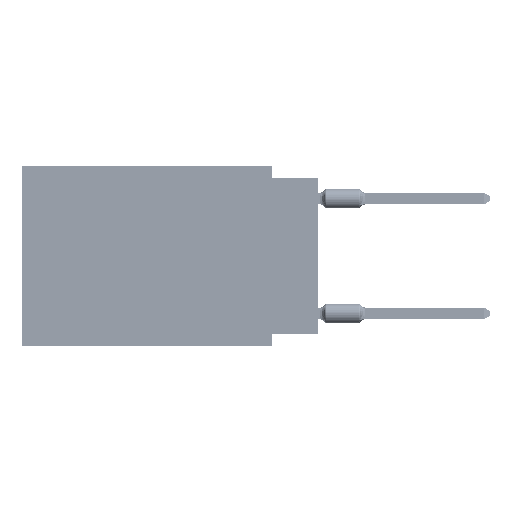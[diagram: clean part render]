
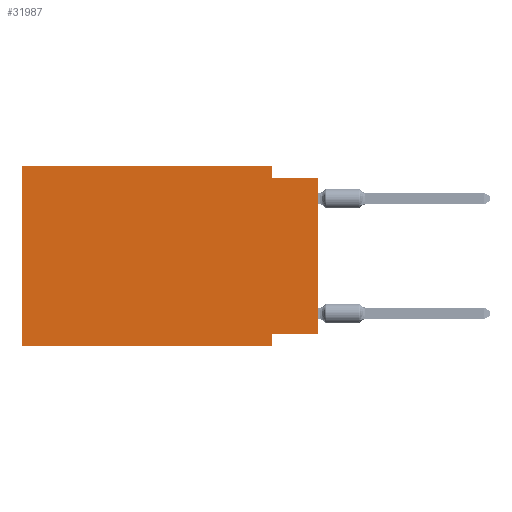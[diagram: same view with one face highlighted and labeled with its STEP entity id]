
A CAD part, left-side view. The second image highlights one B-rep face of the part: STEP entity #31987.
In plain terms, the highlighted planar face has unit normal (-1, 0, 0).
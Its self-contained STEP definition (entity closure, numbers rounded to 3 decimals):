
#2142 = DIRECTION ( 'NONE',  ( 0., 0., -1. ) ) ;
#2933 = LINE ( 'NONE', #9853, #9572 ) ;
#3433 = CARTESIAN_POINT ( 'NONE',  ( 0., 2.54, -9.906 ) ) ;
#5946 = CARTESIAN_POINT ( 'NONE',  ( 0., 0., -9.271 ) ) ;
#6970 = DIRECTION ( 'NONE',  ( 0., -1., 0. ) ) ;
#9033 = VECTOR ( 'NONE', #6970, 1000. ) ;
#9572 = VECTOR ( 'NONE', #56787, 1000. ) ;
#9853 = CARTESIAN_POINT ( 'NONE',  ( 0., 2.54, 0. ) ) ;
#11169 = ORIENTED_EDGE ( 'NONE', *, *, #62654, .F. ) ;
#13111 = VERTEX_POINT ( 'NONE', #47564 ) ;
#13488 = VERTEX_POINT ( 'NONE', #39806 ) ;
#14070 = CARTESIAN_POINT ( 'NONE',  ( 0., 16.383, 0. ) ) ;
#14077 = DIRECTION ( 'NONE',  ( 0., 0., 1. ) ) ;
#14578 = VERTEX_POINT ( 'NONE', #74427 ) ;
#16044 = VECTOR ( 'NONE', #14077, 1000. ) ;
#18585 = DIRECTION ( 'NONE',  ( 0., 0., -1. ) ) ;
#19971 = VECTOR ( 'NONE', #46344, 1000. ) ;
#21335 = VECTOR ( 'NONE', #18585, 1000. ) ;
#21376 = EDGE_CURVE ( 'NONE', #34363, #13488, #2933, .T. ) ;
#21676 = EDGE_LOOP ( 'NONE', ( #48478, #57148, #29792, #11169, #43260, #27646, #43358, #52136 ) ) ;
#22428 = EDGE_CURVE ( 'NONE', #27074, #14578, #39434, .T. ) ;
#22665 = VECTOR ( 'NONE', #39782, 1000. ) ;
#23247 = LINE ( 'NONE', #64027, #19971 ) ;
#24617 = EDGE_CURVE ( 'NONE', #31008, #13111, #66787, .T. ) ;
#26711 = LINE ( 'NONE', #73647, #22665 ) ;
#27074 = VERTEX_POINT ( 'NONE', #58610 ) ;
#27646 = ORIENTED_EDGE ( 'NONE', *, *, #52936, .T. ) ;
#29792 = ORIENTED_EDGE ( 'NONE', *, *, #21376, .F. ) ;
#30497 = LINE ( 'NONE', #3433, #21335 ) ;
#31008 = VERTEX_POINT ( 'NONE', #40539 ) ;
#31987 = ADVANCED_FACE ( 'NONE', ( #43313 ), #55611, .F. ) ;
#34363 = VERTEX_POINT ( 'NONE', #73791 ) ;
#35989 = EDGE_CURVE ( 'NONE', #13488, #38216, #23247, .T. ) ;
#36784 = CARTESIAN_POINT ( 'NONE',  ( 0., 16.383, 0. ) ) ;
#37251 = EDGE_CURVE ( 'NONE', #27074, #38216, #38719, .T. ) ;
#38216 = VERTEX_POINT ( 'NONE', #56623 ) ;
#38719 = LINE ( 'NONE', #67206, #40994 ) ;
#39434 = LINE ( 'NONE', #5946, #74740 ) ;
#39782 = DIRECTION ( 'NONE',  ( 0., -1., 0. ) ) ;
#39806 = CARTESIAN_POINT ( 'NONE',  ( 0., 2.54, -0.635 ) ) ;
#40539 = CARTESIAN_POINT ( 'NONE',  ( 0., 16.383, -9.906 ) ) ;
#40994 = VECTOR ( 'NONE', #55300, 1000. ) ;
#43125 = CARTESIAN_POINT ( 'NONE',  ( 0., 16.383, 0. ) ) ;
#43260 = ORIENTED_EDGE ( 'NONE', *, *, #24617, .F. ) ;
#43313 = FACE_OUTER_BOUND ( 'NONE', #21676, .T. ) ;
#43358 = ORIENTED_EDGE ( 'NONE', *, *, #51948, .F. ) ;
#46344 = DIRECTION ( 'NONE',  ( 0., -1., 0. ) ) ;
#47564 = CARTESIAN_POINT ( 'NONE',  ( 0., 16.383, 0. ) ) ;
#48478 = ORIENTED_EDGE ( 'NONE', *, *, #37251, .T. ) ;
#51948 = EDGE_CURVE ( 'NONE', #14578, #61236, #30497, .T. ) ;
#52136 = ORIENTED_EDGE ( 'NONE', *, *, #22428, .F. ) ;
#52936 = EDGE_CURVE ( 'NONE', #31008, #61236, #26711, .T. ) ;
#54663 = LINE ( 'NONE', #43125, #9033 ) ;
#54858 = DIRECTION ( 'NONE',  ( 1., 0., 0. ) ) ;
#55300 = DIRECTION ( 'NONE',  ( 0., 0., 1. ) ) ;
#55611 = PLANE ( 'NONE',  #60209 ) ;
#56623 = CARTESIAN_POINT ( 'NONE',  ( 0., 0., -0.635 ) ) ;
#56787 = DIRECTION ( 'NONE',  ( 0., 0., -1. ) ) ;
#57148 = ORIENTED_EDGE ( 'NONE', *, *, #35989, .F. ) ;
#58610 = CARTESIAN_POINT ( 'NONE',  ( 0., 0., -9.271 ) ) ;
#59589 = CARTESIAN_POINT ( 'NONE',  ( 0., 2.54, -9.906 ) ) ;
#60209 = AXIS2_PLACEMENT_3D ( 'NONE', #14070, #54858, #2142 ) ;
#61236 = VERTEX_POINT ( 'NONE', #59589 ) ;
#62654 = EDGE_CURVE ( 'NONE', #13111, #34363, #54663, .T. ) ;
#63657 = DIRECTION ( 'NONE',  ( 0., 1., 0. ) ) ;
#64027 = CARTESIAN_POINT ( 'NONE',  ( 0., 0., -0.635 ) ) ;
#66787 = LINE ( 'NONE', #36784, #16044 ) ;
#67206 = CARTESIAN_POINT ( 'NONE',  ( 0., 0., 0. ) ) ;
#73647 = CARTESIAN_POINT ( 'NONE',  ( 0., 16.383, -9.906 ) ) ;
#73791 = CARTESIAN_POINT ( 'NONE',  ( 0., 2.54, 0. ) ) ;
#74427 = CARTESIAN_POINT ( 'NONE',  ( 0., 2.54, -9.271 ) ) ;
#74740 = VECTOR ( 'NONE', #63657, 1000. ) ;
